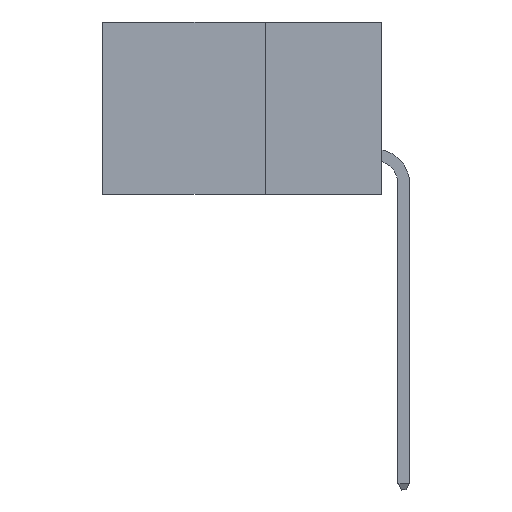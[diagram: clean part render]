
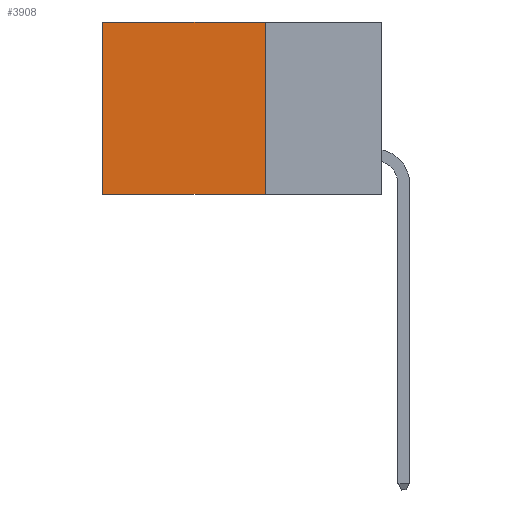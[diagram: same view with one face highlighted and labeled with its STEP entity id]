
A CAD part, left-side view. The second image highlights one B-rep face of the part: STEP entity #3908.
In plain terms, the highlighted planar face has unit normal (-1, 0, 0).
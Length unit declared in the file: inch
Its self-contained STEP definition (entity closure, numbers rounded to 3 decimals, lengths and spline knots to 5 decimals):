
#283 = CARTESIAN_POINT ( 'NONE',  ( 0.2875, 0.6, -0.37 ) ) ;
#402 = CARTESIAN_POINT ( 'NONE',  ( 0.2875, 0.25, 0. ) ) ;
#1056 = AXIS2_PLACEMENT_3D ( 'NONE', #19431, #10530, #15814 ) ;
#2235 = LINE ( 'NONE', #402, #4179 ) ;
#3404 = VERTEX_POINT ( 'NONE', #7292 ) ;
#3606 = LINE ( 'NONE', #5669, #10017 ) ;
#3908 = ADVANCED_FACE ( 'NONE', ( #7033 ), #7025, .F. ) ;
#4025 = ORIENTED_EDGE ( 'NONE', *, *, #17301, .F. ) ;
#4040 = VERTEX_POINT ( 'NONE', #16361 ) ;
#4179 = VECTOR ( 'NONE', #18424, 39.37008 ) ;
#4324 = ORIENTED_EDGE ( 'NONE', *, *, #20742, .F. ) ;
#4487 = EDGE_CURVE ( 'NONE', #3404, #8488, #18136, .T. ) ;
#4533 = CARTESIAN_POINT ( 'NONE',  ( 0.2875, 0.25, -0.37 ) ) ;
#4689 = DIRECTION ( 'NONE',  ( 0., 1., 0. ) ) ;
#5669 = CARTESIAN_POINT ( 'NONE',  ( 0.2875, 0.6, 0. ) ) ;
#7025 = PLANE ( 'NONE',  #1056 ) ;
#7033 = FACE_OUTER_BOUND ( 'NONE', #21940, .T. ) ;
#7292 = CARTESIAN_POINT ( 'NONE',  ( 0.2875, 0.25, 0. ) ) ;
#7389 = ORIENTED_EDGE ( 'NONE', *, *, #21348, .T. ) ;
#8488 = VERTEX_POINT ( 'NONE', #8831 ) ;
#8711 = CARTESIAN_POINT ( 'NONE',  ( 0.2875, 0.25, 0. ) ) ;
#8831 = CARTESIAN_POINT ( 'NONE',  ( 0.2875, 0.6, 0. ) ) ;
#8996 = VECTOR ( 'NONE', #4689, 39.37008 ) ;
#10017 = VECTOR ( 'NONE', #19619, 39.37008 ) ;
#10530 = DIRECTION ( 'NONE',  ( 1., 0., 0. ) ) ;
#13435 = VECTOR ( 'NONE', #13768, 39.37008 ) ;
#13768 = DIRECTION ( 'NONE',  ( 0., 1., 0. ) ) ;
#15814 = DIRECTION ( 'NONE',  ( 0., 0., -1. ) ) ;
#16361 = CARTESIAN_POINT ( 'NONE',  ( 0.2875, 0.25, -0.37 ) ) ;
#17301 = EDGE_CURVE ( 'NONE', #4040, #18575, #17362, .T. ) ;
#17362 = LINE ( 'NONE', #4533, #8996 ) ;
#17490 = ORIENTED_EDGE ( 'NONE', *, *, #4487, .T. ) ;
#18136 = LINE ( 'NONE', #8711, #13435 ) ;
#18424 = DIRECTION ( 'NONE',  ( 0., 0., -1. ) ) ;
#18575 = VERTEX_POINT ( 'NONE', #283 ) ;
#19431 = CARTESIAN_POINT ( 'NONE',  ( 0.2875, 0.25, 0. ) ) ;
#19619 = DIRECTION ( 'NONE',  ( 0., 0., -1. ) ) ;
#20742 = EDGE_CURVE ( 'NONE', #3404, #4040, #2235, .T. ) ;
#21348 = EDGE_CURVE ( 'NONE', #8488, #18575, #3606, .T. ) ;
#21940 = EDGE_LOOP ( 'NONE', ( #7389, #4025, #4324, #17490 ) ) ;
